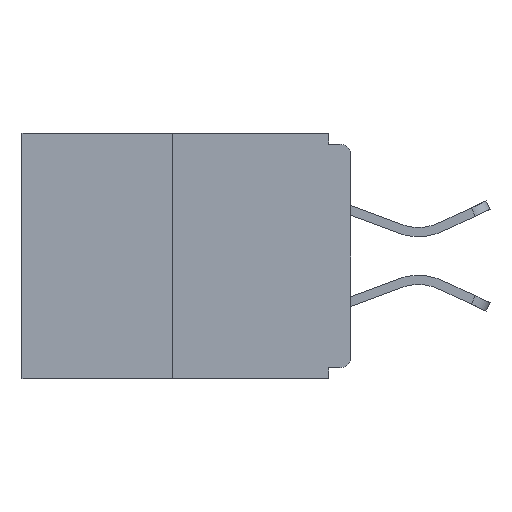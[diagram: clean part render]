
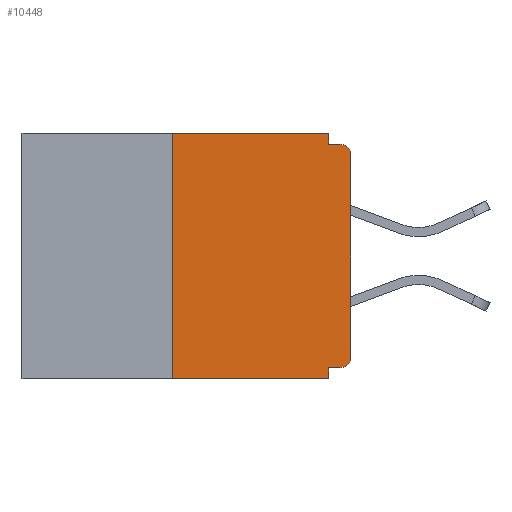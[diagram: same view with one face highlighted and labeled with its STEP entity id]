
A CAD part, left-side view. The second image highlights one B-rep face of the part: STEP entity #10448.
In plain terms, the highlighted planar face has unit normal (-1, 0, 0).
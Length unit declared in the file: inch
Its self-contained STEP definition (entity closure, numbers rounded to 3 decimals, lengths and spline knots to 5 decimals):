
#145 = EDGE_CURVE ( 'NONE', #368, #653, #16513, .T. ) ;
#363 = LINE ( 'NONE', #6410, #4449 ) ;
#368 = VERTEX_POINT ( 'NONE', #7988 ) ;
#511 = CARTESIAN_POINT ( 'NONE',  ( 0., 0.46, 0. ) ) ;
#653 = VERTEX_POINT ( 'NONE', #6704 ) ;
#1012 = LINE ( 'NONE', #10940, #7484 ) ;
#1095 = CARTESIAN_POINT ( 'NONE',  ( 0., 0.015, -0.015 ) ) ;
#1358 = VERTEX_POINT ( 'NONE', #14299 ) ;
#1828 = EDGE_CURVE ( 'NONE', #12216, #4484, #15549, .T. ) ;
#2786 = VERTEX_POINT ( 'NONE', #1095 ) ;
#3373 = ORIENTED_EDGE ( 'NONE', *, *, #7656, .F. ) ;
#3375 = DIRECTION ( 'NONE',  ( 0., 1., 0. ) ) ;
#3453 = ORIENTED_EDGE ( 'NONE', *, *, #1828, .T. ) ;
#3680 = EDGE_CURVE ( 'NONE', #17843, #4298, #5832, .T. ) ;
#3877 = CARTESIAN_POINT ( 'NONE',  ( 0., 0.25, 0. ) ) ;
#4024 = CARTESIAN_POINT ( 'NONE',  ( 0., 0.25, -0.343 ) ) ;
#4228 = CARTESIAN_POINT ( 'NONE',  ( 0., 0.015, -0.328 ) ) ;
#4298 = VERTEX_POINT ( 'NONE', #9078 ) ;
#4449 = VECTOR ( 'NONE', #11609, 39.37008 ) ;
#4463 = AXIS2_PLACEMENT_3D ( 'NONE', #4774, #15754, #15813 ) ;
#4474 = DIRECTION ( 'NONE',  ( 0., 0., -1. ) ) ;
#4484 = VERTEX_POINT ( 'NONE', #13715 ) ;
#4709 = EDGE_CURVE ( 'NONE', #12216, #368, #9876, .T. ) ;
#4774 = CARTESIAN_POINT ( 'NONE',  ( 0., 0.015, -0.313 ) ) ;
#5335 = LINE ( 'NONE', #6827, #17574 ) ;
#5778 = EDGE_CURVE ( 'NONE', #7655, #653, #363, .T. ) ;
#5832 = LINE ( 'NONE', #10018, #9279 ) ;
#6260 = DIRECTION ( 'NONE',  ( 0., -1., 0. ) ) ;
#6410 = CARTESIAN_POINT ( 'NONE',  ( 0., 0.46, -0.343 ) ) ;
#6704 = CARTESIAN_POINT ( 'NONE',  ( 0., 0.031, -0.343 ) ) ;
#6827 = CARTESIAN_POINT ( 'NONE',  ( 0., 0.46, 0. ) ) ;
#6937 = CARTESIAN_POINT ( 'NONE',  ( 0., 0., 0. ) ) ;
#6984 = FACE_OUTER_BOUND ( 'NONE', #11425, .T. ) ;
#7233 = DIRECTION ( 'NONE',  ( 0., 0., -1. ) ) ;
#7277 = ORIENTED_EDGE ( 'NONE', *, *, #9872, .T. ) ;
#7484 = VECTOR ( 'NONE', #11184, 39.37008 ) ;
#7655 = VERTEX_POINT ( 'NONE', #4024 ) ;
#7656 = EDGE_CURVE ( 'NONE', #15629, #17843, #5335, .T. ) ;
#7988 = CARTESIAN_POINT ( 'NONE',  ( 0., 0.031, -0.328 ) ) ;
#8305 = VECTOR ( 'NONE', #6260, 39.37008 ) ;
#8457 = DIRECTION ( 'NONE',  ( -1., 0., 0. ) ) ;
#8709 = VECTOR ( 'NONE', #12478, 39.37008 ) ;
#8802 = VECTOR ( 'NONE', #7233, 39.37008 ) ;
#8910 = ORIENTED_EDGE ( 'NONE', *, *, #145, .F. ) ;
#9078 = CARTESIAN_POINT ( 'NONE',  ( 0., 0.031, -0.015 ) ) ;
#9137 = LINE ( 'NONE', #6937, #8709 ) ;
#9279 = VECTOR ( 'NONE', #11676, 39.37008 ) ;
#9363 = EDGE_CURVE ( 'NONE', #4298, #2786, #13847, .T. ) ;
#9872 = EDGE_CURVE ( 'NONE', #4484, #1358, #9137, .T. ) ;
#9876 = LINE ( 'NONE', #17040, #17612 ) ;
#9878 = AXIS2_PLACEMENT_3D ( 'NONE', #511, #16800, #4474 ) ;
#9883 = ORIENTED_EDGE ( 'NONE', *, *, #5778, .T. ) ;
#10018 = CARTESIAN_POINT ( 'NONE',  ( 0., 0.031, 0. ) ) ;
#10448 = ADVANCED_FACE ( 'NONE', ( #6984 ), #11531, .F. ) ;
#10646 = CARTESIAN_POINT ( 'NONE',  ( 0., 0.031, 0. ) ) ;
#10658 = EDGE_CURVE ( 'NONE', #1358, #2786, #15954, .T. ) ;
#10868 = ORIENTED_EDGE ( 'NONE', *, *, #10658, .T. ) ;
#10940 = CARTESIAN_POINT ( 'NONE',  ( 0., 0.25, 0. ) ) ;
#11184 = DIRECTION ( 'NONE',  ( 0., 0., 1. ) ) ;
#11204 = DIRECTION ( 'NONE',  ( 0., -1., 0. ) ) ;
#11425 = EDGE_LOOP ( 'NONE', ( #3373, #13215, #9883, #8910, #13644, #3453, #7277, #10868, #15253, #11714 ) ) ;
#11531 = PLANE ( 'NONE',  #9878 ) ;
#11609 = DIRECTION ( 'NONE',  ( 0., -1., 0. ) ) ;
#11676 = DIRECTION ( 'NONE',  ( 0., 0., -1. ) ) ;
#11714 = ORIENTED_EDGE ( 'NONE', *, *, #3680, .F. ) ;
#12216 = VERTEX_POINT ( 'NONE', #4228 ) ;
#12478 = DIRECTION ( 'NONE',  ( 0., 0., 1. ) ) ;
#12880 = CARTESIAN_POINT ( 'NONE',  ( 0., 0.031, -0.343 ) ) ;
#13215 = ORIENTED_EDGE ( 'NONE', *, *, #14588, .F. ) ;
#13644 = ORIENTED_EDGE ( 'NONE', *, *, #4709, .F. ) ;
#13699 = DIRECTION ( 'NONE',  ( 0., 0., -1. ) ) ;
#13715 = CARTESIAN_POINT ( 'NONE',  ( 0., 0., -0.313 ) ) ;
#13847 = LINE ( 'NONE', #14562, #8305 ) ;
#14299 = CARTESIAN_POINT ( 'NONE',  ( 0., 0., -0.03 ) ) ;
#14562 = CARTESIAN_POINT ( 'NONE',  ( 0., 0., -0.015 ) ) ;
#14588 = EDGE_CURVE ( 'NONE', #7655, #15629, #1012, .T. ) ;
#15253 = ORIENTED_EDGE ( 'NONE', *, *, #9363, .F. ) ;
#15549 = CIRCLE ( 'NONE', #4463, 0.015 ) ;
#15629 = VERTEX_POINT ( 'NONE', #3877 ) ;
#15754 = DIRECTION ( 'NONE',  ( -1., 0., 0. ) ) ;
#15813 = DIRECTION ( 'NONE',  ( 0., 0., -1. ) ) ;
#15954 = CIRCLE ( 'NONE', #16019, 0.015 ) ;
#16019 = AXIS2_PLACEMENT_3D ( 'NONE', #16464, #8457, #13699 ) ;
#16464 = CARTESIAN_POINT ( 'NONE',  ( 0., 0.015, -0.03 ) ) ;
#16513 = LINE ( 'NONE', #12880, #8802 ) ;
#16800 = DIRECTION ( 'NONE',  ( 1., 0., 0. ) ) ;
#17040 = CARTESIAN_POINT ( 'NONE',  ( 0., 0., -0.328 ) ) ;
#17574 = VECTOR ( 'NONE', #11204, 39.37008 ) ;
#17612 = VECTOR ( 'NONE', #3375, 39.37008 ) ;
#17843 = VERTEX_POINT ( 'NONE', #10646 ) ;
